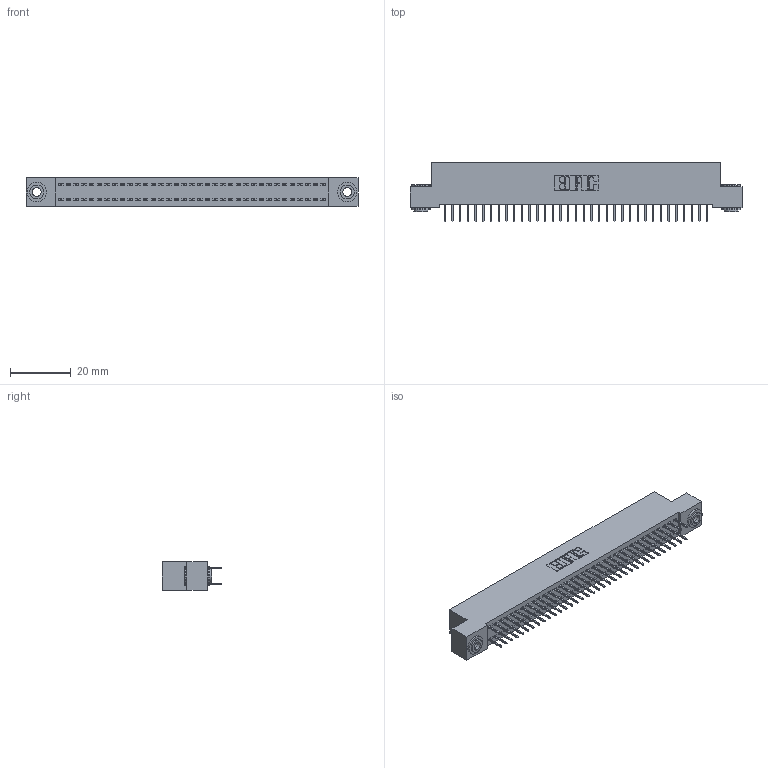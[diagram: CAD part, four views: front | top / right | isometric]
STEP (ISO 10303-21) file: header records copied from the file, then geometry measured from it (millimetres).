
FILE_DESCRIPTION (( 'STEP AP203' ), '1' );
FILE_NAME ('342-070-524-203.STEP', '2019-10-03T15:58:32', ( '' ), ( '' ), 'SwSTEP 2.0', 'SolidWorks 2016', '' );
FILE_SCHEMA (( 'CONFIG_CONTROL_DESIGN' ));
Length unit declared in the file: inch
Products named in the file (4): 342 Part_.156 TH; 345-292-001_345-293-124; 342-250-002_345-250-002-102; 342-070-524-203
Assembly tree (73 placements, depth 2):
  342-070-524-203
    342 Part_.156 TH
    345-292-001_345-293-124  x70
    342-250-002_345-250-002-102  x2
Bounding box: 109.22 x 19.69 x 9.4 mm (x, y, z)
Volume: 9697.2 mm3; surface area: 15550.6 mm2
Topology: 73 solids, 73 shells, 4068 faces, 11505 edges, 7386 vertices
Faces by surface type: plane 3016, cylinder 1044, cone 8
Entity records: 24014 total; most frequent: CARTESIAN_POINT 3961, ORIENTED_EDGE 3890, DIRECTION 3431, EDGE_CURVE 1945, LINE 1797, VECTOR 1797, VERTEX_POINT 1290, AXIS2_PLACEMENT_3D 817
